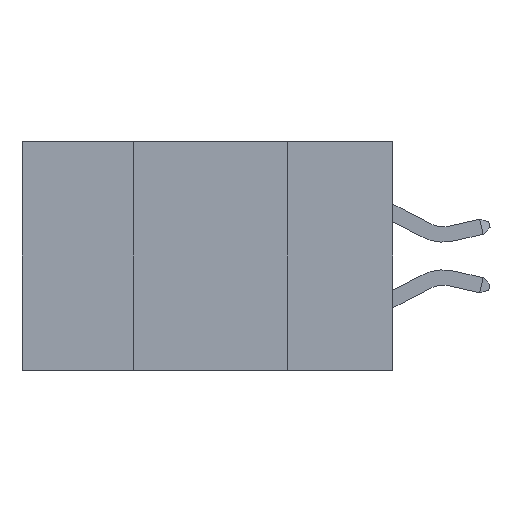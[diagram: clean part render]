
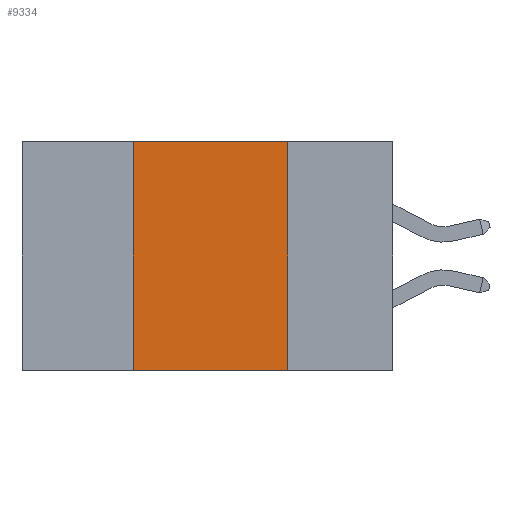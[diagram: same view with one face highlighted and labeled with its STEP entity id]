
A CAD part, left-side view. The second image highlights one B-rep face of the part: STEP entity #9334.
In plain terms, the highlighted planar face has unit normal (-1, 0, 0).
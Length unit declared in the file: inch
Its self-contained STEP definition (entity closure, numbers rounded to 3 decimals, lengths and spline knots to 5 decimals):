
#6 = ORIENTED_EDGE ( 'NONE', *, *, #7162, .T. ) ;
#235 = LINE ( 'NONE', #2890, #9196 ) ;
#340 = DIRECTION ( 'NONE',  ( 0., 0., 1. ) ) ;
#2411 = VERTEX_POINT ( 'NONE', #9865 ) ;
#2463 = EDGE_LOOP ( 'NONE', ( #10076, #5980, #10324, #6 ) ) ;
#2665 = VERTEX_POINT ( 'NONE', #3735 ) ;
#2711 = EDGE_CURVE ( 'NONE', #8630, #8735, #9395, .T. ) ;
#2890 = CARTESIAN_POINT ( 'NONE',  ( 0., 0.17, 0. ) ) ;
#2966 = DIRECTION ( 'NONE',  ( 0., -1., 0. ) ) ;
#3735 = CARTESIAN_POINT ( 'NONE',  ( 0., 0.42, -0.37 ) ) ;
#3840 = CARTESIAN_POINT ( 'NONE',  ( 0., 0.6, -0.37 ) ) ;
#3883 = DIRECTION ( 'NONE',  ( 0., 0., -1. ) ) ;
#4065 = FACE_OUTER_BOUND ( 'NONE', #2463, .T. ) ;
#4066 = AXIS2_PLACEMENT_3D ( 'NONE', #6776, #8784, #10484 ) ;
#4948 = LINE ( 'NONE', #8547, #6012 ) ;
#5035 = CARTESIAN_POINT ( 'NONE',  ( 0., 0.6, 0. ) ) ;
#5065 = EDGE_CURVE ( 'NONE', #2665, #8630, #4948, .T. ) ;
#5094 = VECTOR ( 'NONE', #5791, 39.37008 ) ;
#5791 = DIRECTION ( 'NONE',  ( 0., -1., 0. ) ) ;
#5980 = ORIENTED_EDGE ( 'NONE', *, *, #2711, .F. ) ;
#6012 = VECTOR ( 'NONE', #340, 39.37008 ) ;
#6776 = CARTESIAN_POINT ( 'NONE',  ( 0., 0.6, 0. ) ) ;
#6904 = CARTESIAN_POINT ( 'NONE',  ( 0., 0.17, 0. ) ) ;
#7162 = EDGE_CURVE ( 'NONE', #2665, #2411, #8339, .T. ) ;
#7359 = CARTESIAN_POINT ( 'NONE',  ( 0., 0.42, 0. ) ) ;
#7400 = VECTOR ( 'NONE', #2966, 39.37008 ) ;
#7653 = PLANE ( 'NONE',  #4066 ) ;
#8339 = LINE ( 'NONE', #3840, #7400 ) ;
#8547 = CARTESIAN_POINT ( 'NONE',  ( 0., 0.42, 0. ) ) ;
#8630 = VERTEX_POINT ( 'NONE', #7359 ) ;
#8735 = VERTEX_POINT ( 'NONE', #6904 ) ;
#8784 = DIRECTION ( 'NONE',  ( 1., 0., 0. ) ) ;
#9196 = VECTOR ( 'NONE', #3883, 39.37008 ) ;
#9334 = ADVANCED_FACE ( 'NONE', ( #4065 ), #7653, .F. ) ;
#9395 = LINE ( 'NONE', #5035, #5094 ) ;
#9865 = CARTESIAN_POINT ( 'NONE',  ( 0., 0.17, -0.37 ) ) ;
#10076 = ORIENTED_EDGE ( 'NONE', *, *, #11642, .F. ) ;
#10324 = ORIENTED_EDGE ( 'NONE', *, *, #5065, .F. ) ;
#10484 = DIRECTION ( 'NONE',  ( 0., 0., -1. ) ) ;
#11642 = EDGE_CURVE ( 'NONE', #8735, #2411, #235, .T. ) ;
